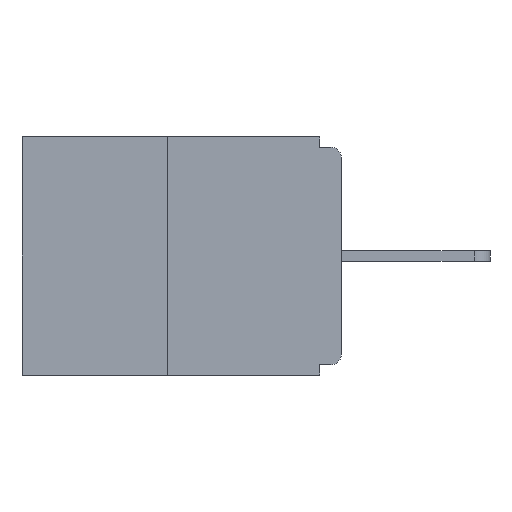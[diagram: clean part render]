
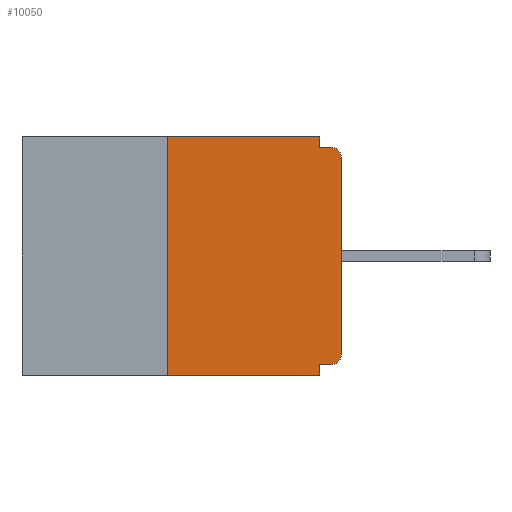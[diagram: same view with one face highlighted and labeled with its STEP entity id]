
A CAD part, left-side view. The second image highlights one B-rep face of the part: STEP entity #10050.
In plain terms, the highlighted planar face has unit normal (-1, 0, 0).
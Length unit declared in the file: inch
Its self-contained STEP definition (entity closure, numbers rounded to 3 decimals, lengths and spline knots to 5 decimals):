
#157 = ORIENTED_EDGE ( 'NONE', *, *, #14561, .F. ) ;
#300 = DIRECTION ( 'NONE',  ( 0., 0., -1. ) ) ;
#324 = ORIENTED_EDGE ( 'NONE', *, *, #10552, .F. ) ;
#734 = DIRECTION ( 'NONE',  ( 0., 0., 1. ) ) ;
#1177 = ORIENTED_EDGE ( 'NONE', *, *, #7339, .F. ) ;
#1563 = AXIS2_PLACEMENT_3D ( 'NONE', #13585, #6547, #14711 ) ;
#1566 = ORIENTED_EDGE ( 'NONE', *, *, #9973, .F. ) ;
#1825 = VERTEX_POINT ( 'NONE', #12648 ) ;
#1978 = VERTEX_POINT ( 'NONE', #3869 ) ;
#2032 = VECTOR ( 'NONE', #2061, 39.37008 ) ;
#2061 = DIRECTION ( 'NONE',  ( 0., -1., 0. ) ) ;
#2557 = CARTESIAN_POINT ( 'NONE',  ( 0., 0., -0.03 ) ) ;
#2692 = VERTEX_POINT ( 'NONE', #5355 ) ;
#3394 = VERTEX_POINT ( 'NONE', #2557 ) ;
#3570 = ORIENTED_EDGE ( 'NONE', *, *, #5075, .T. ) ;
#3869 = CARTESIAN_POINT ( 'NONE',  ( 0., 0.031, -0.343 ) ) ;
#4090 = LINE ( 'NONE', #11535, #12843 ) ;
#4487 = LINE ( 'NONE', #7652, #7380 ) ;
#4493 = CARTESIAN_POINT ( 'NONE',  ( 0., 0., -0.015 ) ) ;
#4543 = DIRECTION ( 'NONE',  ( 0., -1., 0. ) ) ;
#4679 = CARTESIAN_POINT ( 'NONE',  ( 0., 0.015, -0.03 ) ) ;
#4709 = CARTESIAN_POINT ( 'NONE',  ( 0., 0.46, 0. ) ) ;
#4798 = LINE ( 'NONE', #14992, #11224 ) ;
#4823 = CARTESIAN_POINT ( 'NONE',  ( 0., 0.031, 0. ) ) ;
#4834 = LINE ( 'NONE', #15064, #8869 ) ;
#5075 = EDGE_CURVE ( 'NONE', #3394, #8632, #7359, .T. ) ;
#5235 = VECTOR ( 'NONE', #9377, 39.37008 ) ;
#5355 = CARTESIAN_POINT ( 'NONE',  ( 0., 0.031, -0.015 ) ) ;
#5513 = DIRECTION ( 'NONE',  ( 0., 0., 1. ) ) ;
#5588 = EDGE_CURVE ( 'NONE', #7442, #3394, #4090, .T. ) ;
#5672 = CARTESIAN_POINT ( 'NONE',  ( 0., 0.015, -0.328 ) ) ;
#5675 = VERTEX_POINT ( 'NONE', #5672 ) ;
#5912 = DIRECTION ( 'NONE',  ( 0., 0., -1. ) ) ;
#5943 = DIRECTION ( 'NONE',  ( 0., 0., -1. ) ) ;
#6303 = CARTESIAN_POINT ( 'NONE',  ( 0., 0.015, -0.015 ) ) ;
#6547 = DIRECTION ( 'NONE',  ( -1., 0., 0. ) ) ;
#6616 = EDGE_LOOP ( 'NONE', ( #7815, #324, #10055, #7374, #157, #8389, #6992, #3570, #1566, #1177 ) ) ;
#6939 = CARTESIAN_POINT ( 'NONE',  ( 0., 0.46, -0.343 ) ) ;
#6992 = ORIENTED_EDGE ( 'NONE', *, *, #5588, .T. ) ;
#7305 = DIRECTION ( 'NONE',  ( 0., 0., -1. ) ) ;
#7319 = FACE_OUTER_BOUND ( 'NONE', #6616, .T. ) ;
#7339 = EDGE_CURVE ( 'NONE', #7906, #2692, #8740, .T. ) ;
#7359 = CIRCLE ( 'NONE', #13804, 0.015 ) ;
#7374 = ORIENTED_EDGE ( 'NONE', *, *, #8158, .F. ) ;
#7380 = VECTOR ( 'NONE', #300, 39.37008 ) ;
#7442 = VERTEX_POINT ( 'NONE', #13337 ) ;
#7553 = EDGE_CURVE ( 'NONE', #5675, #7442, #14666, .T. ) ;
#7652 = CARTESIAN_POINT ( 'NONE',  ( 0., 0.031, -0.343 ) ) ;
#7815 = ORIENTED_EDGE ( 'NONE', *, *, #14540, .F. ) ;
#7906 = VERTEX_POINT ( 'NONE', #13070 ) ;
#8085 = VECTOR ( 'NONE', #4543, 39.37008 ) ;
#8158 = EDGE_CURVE ( 'NONE', #1825, #1978, #4487, .T. ) ;
#8163 = DIRECTION ( 'NONE',  ( 0., 1., 0. ) ) ;
#8389 = ORIENTED_EDGE ( 'NONE', *, *, #7553, .T. ) ;
#8475 = LINE ( 'NONE', #4493, #8085 ) ;
#8632 = VERTEX_POINT ( 'NONE', #6303 ) ;
#8740 = LINE ( 'NONE', #4823, #11823 ) ;
#8757 = CARTESIAN_POINT ( 'NONE',  ( 0., 0.25, 0. ) ) ;
#8869 = VECTOR ( 'NONE', #8163, 39.37008 ) ;
#8975 = EDGE_CURVE ( 'NONE', #12051, #1978, #11604, .T. ) ;
#9320 = CARTESIAN_POINT ( 'NONE',  ( 0., 0.46, 0. ) ) ;
#9377 = DIRECTION ( 'NONE',  ( 0., -1., 0. ) ) ;
#9706 = CARTESIAN_POINT ( 'NONE',  ( 0., 0.25, -0.343 ) ) ;
#9973 = EDGE_CURVE ( 'NONE', #2692, #8632, #8475, .T. ) ;
#10050 = ADVANCED_FACE ( 'NONE', ( #7319 ), #11876, .F. ) ;
#10055 = ORIENTED_EDGE ( 'NONE', *, *, #8975, .T. ) ;
#10552 = EDGE_CURVE ( 'NONE', #12051, #14226, #4798, .T. ) ;
#11224 = VECTOR ( 'NONE', #734, 39.37008 ) ;
#11287 = AXIS2_PLACEMENT_3D ( 'NONE', #4709, #13032, #5943 ) ;
#11535 = CARTESIAN_POINT ( 'NONE',  ( 0., 0., 0. ) ) ;
#11604 = LINE ( 'NONE', #6939, #5235 ) ;
#11823 = VECTOR ( 'NONE', #7305, 39.37008 ) ;
#11876 = PLANE ( 'NONE',  #11287 ) ;
#12051 = VERTEX_POINT ( 'NONE', #9706 ) ;
#12648 = CARTESIAN_POINT ( 'NONE',  ( 0., 0.031, -0.328 ) ) ;
#12843 = VECTOR ( 'NONE', #5513, 39.37008 ) ;
#13000 = DIRECTION ( 'NONE',  ( -1., 0., 0. ) ) ;
#13032 = DIRECTION ( 'NONE',  ( 1., 0., 0. ) ) ;
#13070 = CARTESIAN_POINT ( 'NONE',  ( 0., 0.031, 0. ) ) ;
#13337 = CARTESIAN_POINT ( 'NONE',  ( 0., 0., -0.313 ) ) ;
#13585 = CARTESIAN_POINT ( 'NONE',  ( 0., 0.015, -0.313 ) ) ;
#13804 = AXIS2_PLACEMENT_3D ( 'NONE', #4679, #13000, #5912 ) ;
#14226 = VERTEX_POINT ( 'NONE', #8757 ) ;
#14271 = LINE ( 'NONE', #9320, #2032 ) ;
#14540 = EDGE_CURVE ( 'NONE', #14226, #7906, #14271, .T. ) ;
#14561 = EDGE_CURVE ( 'NONE', #5675, #1825, #4834, .T. ) ;
#14666 = CIRCLE ( 'NONE', #1563, 0.015 ) ;
#14711 = DIRECTION ( 'NONE',  ( 0., 0., -1. ) ) ;
#14992 = CARTESIAN_POINT ( 'NONE',  ( 0., 0.25, 0. ) ) ;
#15064 = CARTESIAN_POINT ( 'NONE',  ( 0., 0., -0.328 ) ) ;
